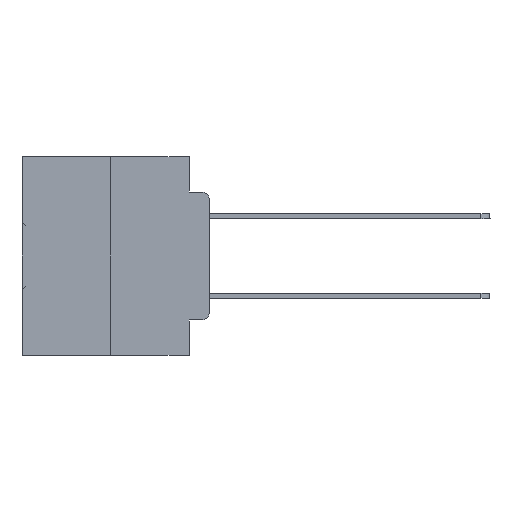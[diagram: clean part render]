
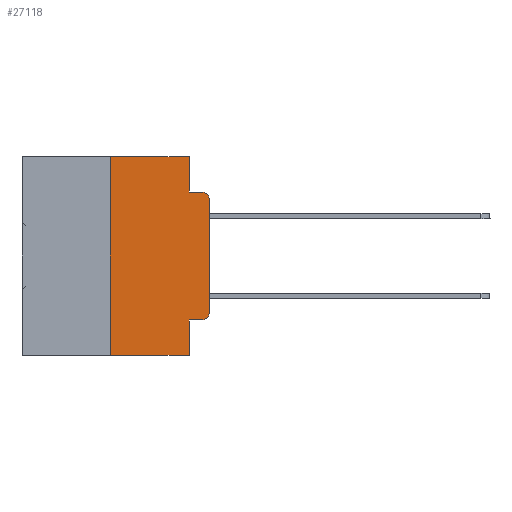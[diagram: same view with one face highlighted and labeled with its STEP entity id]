
A CAD part, left-side view. The second image highlights one B-rep face of the part: STEP entity #27118.
In plain terms, the highlighted planar face has unit normal (-1, 0, 0).
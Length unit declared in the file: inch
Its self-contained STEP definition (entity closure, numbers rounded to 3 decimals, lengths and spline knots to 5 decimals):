
#484 = DIRECTION ( 'NONE',  ( 0., 0., 1. ) ) ;
#1122 = AXIS2_PLACEMENT_3D ( 'NONE', #9819, #30266, #12803 ) ;
#1127 = AXIS2_PLACEMENT_3D ( 'NONE', #12703, #33043, #15650 ) ;
#2081 = VERTEX_POINT ( 'NONE', #5072 ) ;
#3106 = EDGE_CURVE ( 'NONE', #8576, #2081, #5086, .T. ) ;
#3412 = CARTESIAN_POINT ( 'NONE',  ( 0., 0.25, -0.5 ) ) ;
#4728 = LINE ( 'NONE', #14289, #19445 ) ;
#4809 = CIRCLE ( 'NONE', #1122, 0.02 ) ;
#5072 = CARTESIAN_POINT ( 'NONE',  ( 0., 0.25, 0. ) ) ;
#5086 = LINE ( 'NONE', #16965, #26620 ) ;
#5094 = EDGE_CURVE ( 'NONE', #22337, #19725, #31941, .T. ) ;
#5256 = ORIENTED_EDGE ( 'NONE', *, *, #15450, .T. ) ;
#5529 = DIRECTION ( 'NONE',  ( 0., -1., 0. ) ) ;
#5782 = DIRECTION ( 'NONE',  ( 0., 0., -1. ) ) ;
#6696 = ORIENTED_EDGE ( 'NONE', *, *, #12995, .T. ) ;
#6968 = LINE ( 'NONE', #27622, #36073 ) ;
#7071 = EDGE_CURVE ( 'NONE', #19725, #20850, #11418, .T. ) ;
#7650 = DIRECTION ( 'NONE',  ( 0., -1., 0. ) ) ;
#7670 = FACE_OUTER_BOUND ( 'NONE', #26340, .T. ) ;
#7805 = CARTESIAN_POINT ( 'NONE',  ( 0., 0.051, -0.0885 ) ) ;
#8576 = VERTEX_POINT ( 'NONE', #3412 ) ;
#8765 = ORIENTED_EDGE ( 'NONE', *, *, #33196, .T. ) ;
#8787 = CARTESIAN_POINT ( 'NONE',  ( 0., 0.051, -0.0885 ) ) ;
#9819 = CARTESIAN_POINT ( 'NONE',  ( 0., 0.02, -0.3915 ) ) ;
#9937 = VERTEX_POINT ( 'NONE', #21321 ) ;
#10022 = VECTOR ( 'NONE', #22949, 39.37008 ) ;
#10139 = CARTESIAN_POINT ( 'NONE',  ( 0., 0., -0.3915 ) ) ;
#10485 = VECTOR ( 'NONE', #7650, 39.37008 ) ;
#11053 = CARTESIAN_POINT ( 'NONE',  ( 0., 0.051, 0. ) ) ;
#11078 = DIRECTION ( 'NONE',  ( 1., 0., 0. ) ) ;
#11224 = ORIENTED_EDGE ( 'NONE', *, *, #30129, .F. ) ;
#11418 = LINE ( 'NONE', #8787, #10485 ) ;
#11425 = CARTESIAN_POINT ( 'NONE',  ( 0., 0.473, -0.5 ) ) ;
#12117 = CIRCLE ( 'NONE', #1127, 0.02 ) ;
#12504 = ORIENTED_EDGE ( 'NONE', *, *, #14968, .T. ) ;
#12577 = CARTESIAN_POINT ( 'NONE',  ( 0., 0., -0.1085 ) ) ;
#12703 = CARTESIAN_POINT ( 'NONE',  ( 0., 0.02, -0.1085 ) ) ;
#12803 = DIRECTION ( 'NONE',  ( 0., 0., -1. ) ) ;
#12941 = VECTOR ( 'NONE', #484, 39.37008 ) ;
#12995 = EDGE_CURVE ( 'NONE', #32513, #20850, #12117, .T. ) ;
#13890 = DIRECTION ( 'NONE',  ( 0., 0., 1. ) ) ;
#14289 = CARTESIAN_POINT ( 'NONE',  ( 0., 0.473, 0. ) ) ;
#14968 = EDGE_CURVE ( 'NONE', #16354, #32513, #20731, .T. ) ;
#15450 = EDGE_CURVE ( 'NONE', #8576, #24744, #35144, .T. ) ;
#15650 = DIRECTION ( 'NONE',  ( 0., 0., -1. ) ) ;
#16257 = VERTEX_POINT ( 'NONE', #20870 ) ;
#16354 = VERTEX_POINT ( 'NONE', #10139 ) ;
#16474 = CARTESIAN_POINT ( 'NONE',  ( 0., 0.02, -0.0885 ) ) ;
#16965 = CARTESIAN_POINT ( 'NONE',  ( 0., 0.25, 0. ) ) ;
#17413 = VECTOR ( 'NONE', #5782, 39.37008 ) ;
#18182 = CARTESIAN_POINT ( 'NONE',  ( 0., 0.051, 0. ) ) ;
#19074 = ORIENTED_EDGE ( 'NONE', *, *, #3106, .F. ) ;
#19445 = VECTOR ( 'NONE', #5529, 39.37008 ) ;
#19725 = VERTEX_POINT ( 'NONE', #7805 ) ;
#20731 = LINE ( 'NONE', #35464, #12941 ) ;
#20850 = VERTEX_POINT ( 'NONE', #16474 ) ;
#20870 = CARTESIAN_POINT ( 'NONE',  ( 0., 0.051, -0.4115 ) ) ;
#21156 = ORIENTED_EDGE ( 'NONE', *, *, #35111, .F. ) ;
#21321 = CARTESIAN_POINT ( 'NONE',  ( 0., 0.02, -0.4115 ) ) ;
#22337 = VERTEX_POINT ( 'NONE', #11053 ) ;
#22342 = CARTESIAN_POINT ( 'NONE',  ( 0., 0.051, -0.5 ) ) ;
#22778 = CARTESIAN_POINT ( 'NONE',  ( 0., 0.473, 0. ) ) ;
#22949 = DIRECTION ( 'NONE',  ( 0., 0., -1. ) ) ;
#24744 = VERTEX_POINT ( 'NONE', #22342 ) ;
#25611 = LINE ( 'NONE', #37240, #10022 ) ;
#26340 = EDGE_LOOP ( 'NONE', ( #12504, #6696, #31374, #31038, #11224, #19074, #5256, #21156, #8765, #30251 ) ) ;
#26599 = VECTOR ( 'NONE', #28826, 39.37008 ) ;
#26620 = VECTOR ( 'NONE', #13890, 39.37008 ) ;
#27118 = ADVANCED_FACE ( 'NONE', ( #7670 ), #28628, .F. ) ;
#27622 = CARTESIAN_POINT ( 'NONE',  ( 0., 0.051, -0.4115 ) ) ;
#28562 = AXIS2_PLACEMENT_3D ( 'NONE', #22778, #11078, #31487 ) ;
#28628 = PLANE ( 'NONE',  #28562 ) ;
#28826 = DIRECTION ( 'NONE',  ( 0., -1., 0. ) ) ;
#30129 = EDGE_CURVE ( 'NONE', #2081, #22337, #4728, .T. ) ;
#30251 = ORIENTED_EDGE ( 'NONE', *, *, #31278, .T. ) ;
#30266 = DIRECTION ( 'NONE',  ( -1., 0., 0. ) ) ;
#30504 = DIRECTION ( 'NONE',  ( 0., -1., 0. ) ) ;
#31038 = ORIENTED_EDGE ( 'NONE', *, *, #5094, .F. ) ;
#31278 = EDGE_CURVE ( 'NONE', #9937, #16354, #4809, .T. ) ;
#31374 = ORIENTED_EDGE ( 'NONE', *, *, #7071, .F. ) ;
#31487 = DIRECTION ( 'NONE',  ( 0., 0., -1. ) ) ;
#31941 = LINE ( 'NONE', #18182, #17413 ) ;
#32513 = VERTEX_POINT ( 'NONE', #12577 ) ;
#33043 = DIRECTION ( 'NONE',  ( -1., 0., 0. ) ) ;
#33196 = EDGE_CURVE ( 'NONE', #16257, #9937, #6968, .T. ) ;
#35111 = EDGE_CURVE ( 'NONE', #16257, #24744, #25611, .T. ) ;
#35144 = LINE ( 'NONE', #11425, #26599 ) ;
#35464 = CARTESIAN_POINT ( 'NONE',  ( 0., 0., 0. ) ) ;
#36073 = VECTOR ( 'NONE', #30504, 39.37008 ) ;
#37240 = CARTESIAN_POINT ( 'NONE',  ( 0., 0.051, 0. ) ) ;
